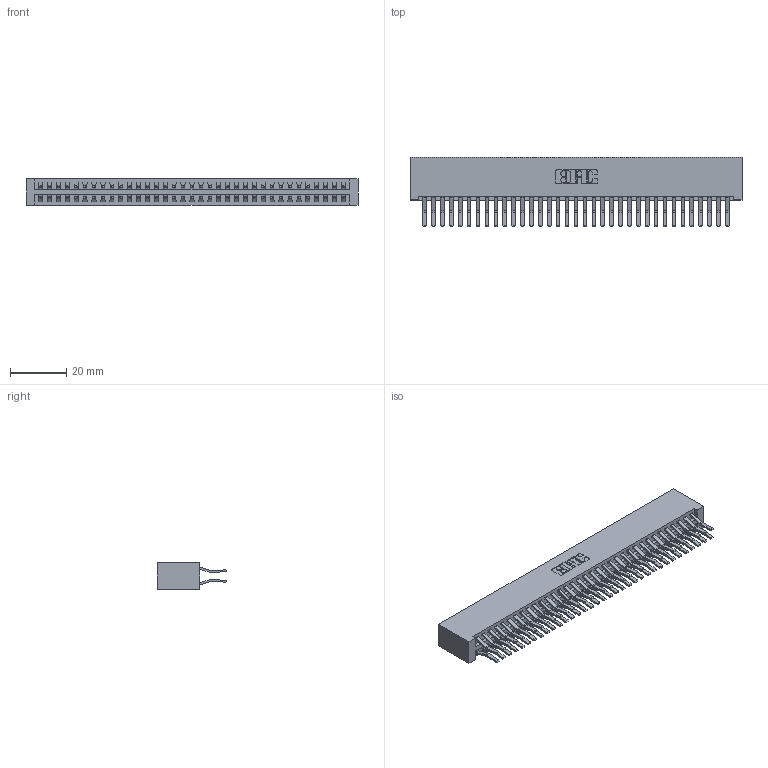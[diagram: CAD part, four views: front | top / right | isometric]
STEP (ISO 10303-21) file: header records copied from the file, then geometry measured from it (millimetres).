
FILE_DESCRIPTION (( 'STEP AP203' ), '1' );
FILE_NAME ('346-070-560-201.STEP', '2022-05-24T22:38:48', ( '' ), ( '' ), 'SwSTEP 2.0', 'SolidWorks 2020', '' );
FILE_SCHEMA (( 'CONFIG_CONTROL_DESIGN' ));
Length unit declared in the file: inch
Products named in the file (3): 346-070-560-201; 345-292-001_560 Tail; 346 Part_No Mounting Lugs
Assembly tree (71 placements, depth 2):
  346-070-560-201
    346 Part_No Mounting Lugs
    345-292-001_560 Tail  x70
Bounding box: 118.36 x 24.78 x 9.4 mm (x, y, z)
Volume: 12519.7 mm3; surface area: 18486.4 mm2
Topology: 71 solids, 71 shells, 3894 faces, 11575 edges, 7622 vertices
Faces by surface type: plane 2522, cylinder 1372
Entity records: 23595 total; most frequent: CARTESIAN_POINT 3896, ORIENTED_EDGE 3830, DIRECTION 3483, EDGE_CURVE 1915, LINE 1647, VECTOR 1647, VERTEX_POINT 1274, AXIS2_PLACEMENT_3D 918
